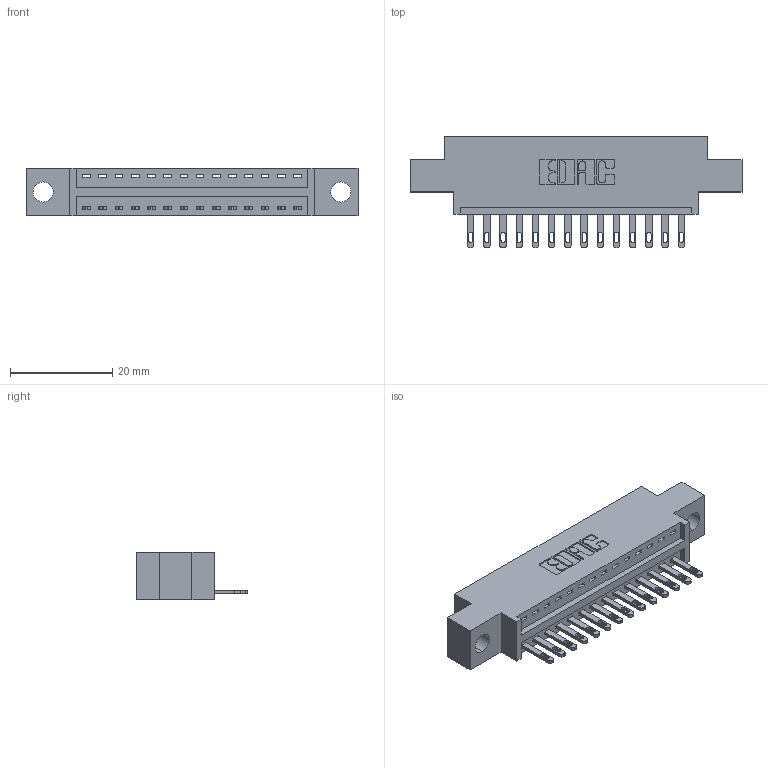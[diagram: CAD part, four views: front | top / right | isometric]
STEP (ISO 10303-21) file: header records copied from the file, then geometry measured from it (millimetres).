
FILE_DESCRIPTION (( 'STEP AP203' ), '1' );
FILE_NAME ('346-014-500-604.STEP', '2022-05-05T05:33:29', ( '' ), ( '' ), 'SwSTEP 2.0', 'SolidWorks 2020', '' );
FILE_SCHEMA (( 'CONFIG_CONTROL_DESIGN' ));
Length unit declared in the file: inch
Products named in the file (3): 346-014-500-604; 345-292-001_345-293-100; 346 Part_0.170 Offset - 0.156 Dia-TH
Assembly tree (15 placements, depth 2):
  346-014-500-604
    346 Part_0.170 Offset - 0.156 Dia-TH
    345-292-001_345-293-100  x14
Bounding box: 65.02 x 21.84 x 9.4 mm (x, y, z)
Volume: 5779.4 mm3; surface area: 6951.6 mm2
Topology: 15 solids, 15 shells, 896 faces, 2729 edges, 1818 vertices
Faces by surface type: plane 570, cylinder 326
Entity records: 12939 total; most frequent: CARTESIAN_POINT 2236, ORIENTED_EDGE 2182, DIRECTION 2007, EDGE_CURVE 1091, VECTOR 899, LINE 899, VERTEX_POINT 726, AXIS2_PLACEMENT_3D 554
